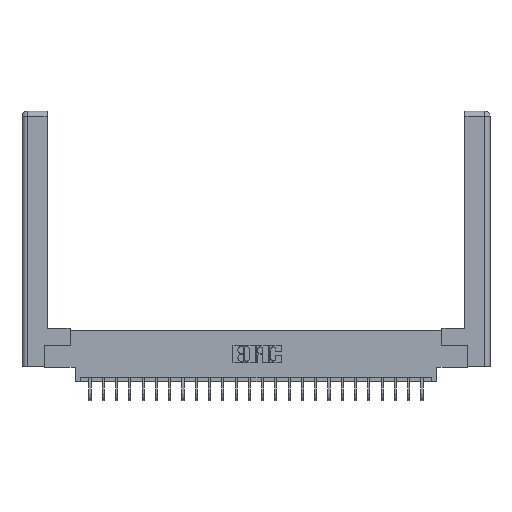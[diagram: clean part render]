
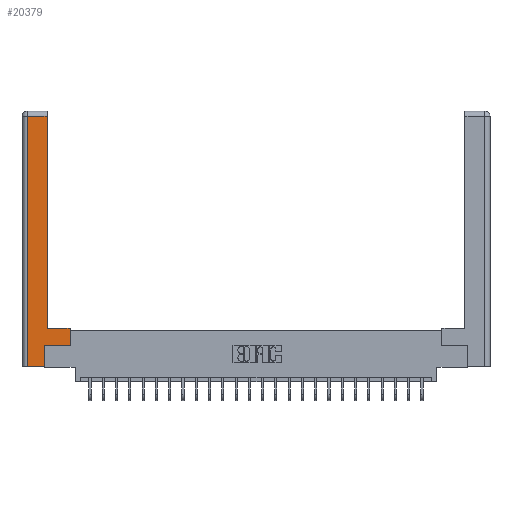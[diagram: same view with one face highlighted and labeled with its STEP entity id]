
A CAD part, top view. The second image highlights one B-rep face of the part: STEP entity #20379.
In plain terms, the highlighted planar face has unit normal (0, 0, 1).
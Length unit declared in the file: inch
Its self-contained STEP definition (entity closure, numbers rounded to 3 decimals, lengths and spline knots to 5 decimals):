
#43 = DIRECTION ( 'NONE',  ( 0., 1., 0. ) ) ;
#675 = CARTESIAN_POINT ( 'NONE',  ( 0.265, 0.245, 0. ) ) ;
#737 = CARTESIAN_POINT ( 'NONE',  ( 0.565, 0.45, 0. ) ) ;
#1178 = ORIENTED_EDGE ( 'NONE', *, *, #21874, .T. ) ;
#1443 = CARTESIAN_POINT ( 'NONE',  ( 0.295, 0.45, 0. ) ) ;
#2054 = DIRECTION ( 'NONE',  ( 0., 1., 0. ) ) ;
#3057 = VECTOR ( 'NONE', #15933, 39.37008 ) ;
#3080 = VERTEX_POINT ( 'NONE', #22955 ) ;
#3195 = ORIENTED_EDGE ( 'NONE', *, *, #25455, .T. ) ;
#3245 = LINE ( 'NONE', #13981, #5898 ) ;
#4750 = CARTESIAN_POINT ( 'NONE',  ( 0.295, 2.94, 0. ) ) ;
#4762 = DIRECTION ( 'NONE',  ( 0., -1., 0. ) ) ;
#5412 = VECTOR ( 'NONE', #4762, 39.37008 ) ;
#5898 = VECTOR ( 'NONE', #24061, 39.37008 ) ;
#6591 = VECTOR ( 'NONE', #20299, 39.37008 ) ;
#7267 = FACE_OUTER_BOUND ( 'NONE', #15691, .T. ) ;
#7305 = VERTEX_POINT ( 'NONE', #737 ) ;
#7461 = PLANE ( 'NONE',  #8302 ) ;
#7571 = VECTOR ( 'NONE', #26394, 39.37008 ) ;
#7965 = LINE ( 'NONE', #1443, #3057 ) ;
#8302 = AXIS2_PLACEMENT_3D ( 'NONE', #9542, #15585, #25764 ) ;
#9106 = EDGE_CURVE ( 'NONE', #3080, #17191, #25444, .T. ) ;
#9477 = LINE ( 'NONE', #24907, #23365 ) ;
#9542 = CARTESIAN_POINT ( 'NONE',  ( 0., 0., 0. ) ) ;
#10719 = CARTESIAN_POINT ( 'NONE',  ( 0.265, 0., 0. ) ) ;
#10933 = EDGE_CURVE ( 'NONE', #16988, #13987, #3245, .T. ) ;
#10957 = ORIENTED_EDGE ( 'NONE', *, *, #25286, .T. ) ;
#13599 = CARTESIAN_POINT ( 'NONE',  ( 0.0615, 2.94, 0. ) ) ;
#13981 = CARTESIAN_POINT ( 'NONE',  ( 0.565, 0.245, 0. ) ) ;
#13987 = VERTEX_POINT ( 'NONE', #15433 ) ;
#14694 = VECTOR ( 'NONE', #2054, 39.37008 ) ;
#15135 = CARTESIAN_POINT ( 'NONE',  ( 0.0615, 0., 0. ) ) ;
#15181 = VERTEX_POINT ( 'NONE', #16848 ) ;
#15433 = CARTESIAN_POINT ( 'NONE',  ( 0.565, 0.245, 0. ) ) ;
#15585 = DIRECTION ( 'NONE',  ( 0., 0., -1. ) ) ;
#15691 = EDGE_LOOP ( 'NONE', ( #16027, #22286, #18898, #3195, #23999, #18370, #10957, #1178 ) ) ;
#15933 = DIRECTION ( 'NONE',  ( -1., 0., 0. ) ) ;
#16027 = ORIENTED_EDGE ( 'NONE', *, *, #20506, .T. ) ;
#16848 = CARTESIAN_POINT ( 'NONE',  ( 0.295, 0.45, 0. ) ) ;
#16988 = VERTEX_POINT ( 'NONE', #675 ) ;
#17038 = DIRECTION ( 'NONE',  ( 1., 0., 0. ) ) ;
#17132 = CARTESIAN_POINT ( 'NONE',  ( 0.0615, 0., 0. ) ) ;
#17191 = VERTEX_POINT ( 'NONE', #15135 ) ;
#17492 = VECTOR ( 'NONE', #17038, 39.37008 ) ;
#18370 = ORIENTED_EDGE ( 'NONE', *, *, #10933, .T. ) ;
#18715 = VERTEX_POINT ( 'NONE', #10719 ) ;
#18898 = ORIENTED_EDGE ( 'NONE', *, *, #9106, .T. ) ;
#19036 = CARTESIAN_POINT ( 'NONE',  ( 0.265, 0., 0. ) ) ;
#19453 = LINE ( 'NONE', #19036, #17492 ) ;
#20067 = CARTESIAN_POINT ( 'NONE',  ( 0.295, 3., 0. ) ) ;
#20299 = DIRECTION ( 'NONE',  ( -1., 0., 0. ) ) ;
#20379 = ADVANCED_FACE ( 'NONE', ( #7267 ), #7461, .F. ) ;
#20506 = EDGE_CURVE ( 'NONE', #15181, #22905, #22430, .T. ) ;
#21874 = EDGE_CURVE ( 'NONE', #7305, #15181, #7965, .T. ) ;
#22286 = ORIENTED_EDGE ( 'NONE', *, *, #25056, .T. ) ;
#22430 = LINE ( 'NONE', #20067, #7571 ) ;
#22905 = VERTEX_POINT ( 'NONE', #4750 ) ;
#22955 = CARTESIAN_POINT ( 'NONE',  ( 0.0615, 2.94, 0. ) ) ;
#23365 = VECTOR ( 'NONE', #43, 39.37008 ) ;
#23999 = ORIENTED_EDGE ( 'NONE', *, *, #24582, .T. ) ;
#24061 = DIRECTION ( 'NONE',  ( 1., 0., 0. ) ) ;
#24582 = EDGE_CURVE ( 'NONE', #18715, #16988, #26279, .T. ) ;
#24803 = CARTESIAN_POINT ( 'NONE',  ( 0.265, 0.245, 0. ) ) ;
#24907 = CARTESIAN_POINT ( 'NONE',  ( 0.565, 0.45, 0. ) ) ;
#25056 = EDGE_CURVE ( 'NONE', #22905, #3080, #26573, .T. ) ;
#25286 = EDGE_CURVE ( 'NONE', #13987, #7305, #9477, .T. ) ;
#25444 = LINE ( 'NONE', #17132, #5412 ) ;
#25455 = EDGE_CURVE ( 'NONE', #17191, #18715, #19453, .T. ) ;
#25764 = DIRECTION ( 'NONE',  ( -1., 0., 0. ) ) ;
#26279 = LINE ( 'NONE', #24803, #14694 ) ;
#26394 = DIRECTION ( 'NONE',  ( 0., 1., 0. ) ) ;
#26573 = LINE ( 'NONE', #13599, #6591 ) ;
